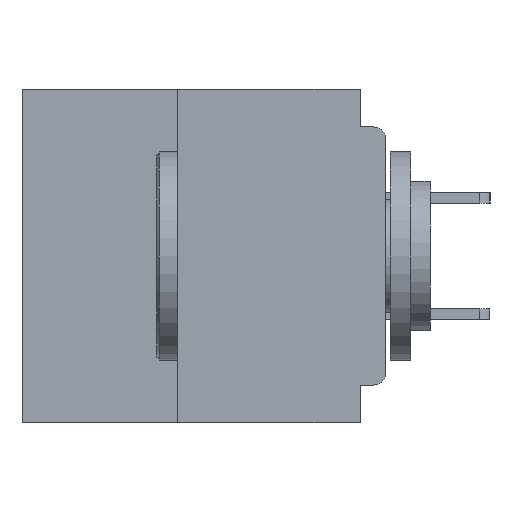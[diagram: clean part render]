
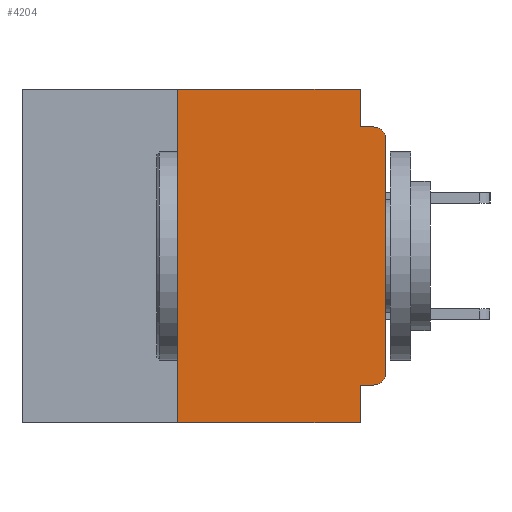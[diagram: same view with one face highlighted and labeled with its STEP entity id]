
A CAD part, left-side view. The second image highlights one B-rep face of the part: STEP entity #4204.
In plain terms, the highlighted planar face has unit normal (-1, 0, 0).
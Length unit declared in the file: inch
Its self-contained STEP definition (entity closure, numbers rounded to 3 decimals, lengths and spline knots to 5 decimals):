
#66 = VECTOR ( 'NONE', #5726, 39.37008 ) ;
#477 = ORIENTED_EDGE ( 'NONE', *, *, #27750, .T. ) ;
#1246 = LINE ( 'NONE', #16728, #11115 ) ;
#1715 = DIRECTION ( 'NONE',  ( 0., 0., -1. ) ) ;
#1983 = CARTESIAN_POINT ( 'NONE',  ( 0., 0., -0.045 ) ) ;
#2446 = CARTESIAN_POINT ( 'NONE',  ( 0., 0.015, -0.34 ) ) ;
#2610 = PLANE ( 'NONE',  #32171 ) ;
#2811 = EDGE_CURVE ( 'NONE', #2986, #11895, #3946, .T. ) ;
#2986 = VERTEX_POINT ( 'NONE', #45471 ) ;
#3946 = LINE ( 'NONE', #13473, #12645 ) ;
#3981 = ORIENTED_EDGE ( 'NONE', *, *, #2811, .F. ) ;
#4070 = CIRCLE ( 'NONE', #30709, 0.015 ) ;
#4204 = ADVANCED_FACE ( 'NONE', ( #39457 ), #2610, .F. ) ;
#5159 = ORIENTED_EDGE ( 'NONE', *, *, #5538, .F. ) ;
#5538 = EDGE_CURVE ( 'NONE', #42460, #2986, #29608, .T. ) ;
#5726 = DIRECTION ( 'NONE',  ( 0., -1., 0. ) ) ;
#6201 = DIRECTION ( 'NONE',  ( 0., 0., -1. ) ) ;
#6275 = ORIENTED_EDGE ( 'NONE', *, *, #23283, .F. ) ;
#6355 = DIRECTION ( 'NONE',  ( 1., 0., 0. ) ) ;
#6755 = EDGE_CURVE ( 'NONE', #13888, #23296, #25485, .T. ) ;
#8446 = LINE ( 'NONE', #23642, #26882 ) ;
#10859 = ORIENTED_EDGE ( 'NONE', *, *, #11515, .F. ) ;
#11115 = VECTOR ( 'NONE', #35025, 39.37008 ) ;
#11515 = EDGE_CURVE ( 'NONE', #15587, #40339, #39243, .T. ) ;
#11659 = DIRECTION ( 'NONE',  ( 0., 0., -1. ) ) ;
#11895 = VERTEX_POINT ( 'NONE', #29669 ) ;
#12645 = VECTOR ( 'NONE', #11659, 39.37008 ) ;
#12941 = VECTOR ( 'NONE', #17862, 39.37008 ) ;
#13473 = CARTESIAN_POINT ( 'NONE',  ( 0., 0.031, -0.4 ) ) ;
#13888 = VERTEX_POINT ( 'NONE', #44891 ) ;
#14512 = EDGE_CURVE ( 'NONE', #21854, #15587, #8446, .T. ) ;
#15587 = VERTEX_POINT ( 'NONE', #29735 ) ;
#16728 = CARTESIAN_POINT ( 'NONE',  ( 0., 0.25, -0.4 ) ) ;
#17862 = DIRECTION ( 'NONE',  ( 0., -1., 0. ) ) ;
#18737 = VECTOR ( 'NONE', #28932, 39.37008 ) ;
#21364 = VECTOR ( 'NONE', #36118, 39.37008 ) ;
#21854 = VERTEX_POINT ( 'NONE', #30813 ) ;
#21894 = VERTEX_POINT ( 'NONE', #45613 ) ;
#21908 = ORIENTED_EDGE ( 'NONE', *, *, #47481, .F. ) ;
#22548 = ORIENTED_EDGE ( 'NONE', *, *, #40474, .T. ) ;
#23283 = EDGE_CURVE ( 'NONE', #21894, #21854, #23938, .T. ) ;
#23296 = VERTEX_POINT ( 'NONE', #29077 ) ;
#23639 = CARTESIAN_POINT ( 'NONE',  ( 0., 0.25, -0.4 ) ) ;
#23642 = CARTESIAN_POINT ( 'NONE',  ( 0., 0.031, 0. ) ) ;
#23883 = DIRECTION ( 'NONE',  ( -1., 0., 0. ) ) ;
#23938 = LINE ( 'NONE', #47072, #12941 ) ;
#24154 = ORIENTED_EDGE ( 'NONE', *, *, #14512, .F. ) ;
#24997 = CARTESIAN_POINT ( 'NONE',  ( 0., 0., 0. ) ) ;
#25485 = LINE ( 'NONE', #24997, #43751 ) ;
#25825 = ORIENTED_EDGE ( 'NONE', *, *, #6755, .T. ) ;
#26882 = VECTOR ( 'NONE', #45294, 39.37008 ) ;
#27337 = EDGE_CURVE ( 'NONE', #23296, #40339, #30491, .T. ) ;
#27750 = EDGE_CURVE ( 'NONE', #42325, #11895, #40779, .T. ) ;
#28062 = CARTESIAN_POINT ( 'NONE',  ( 0., 0.015, -0.355 ) ) ;
#28242 = DIRECTION ( 'NONE',  ( -1., 0., 0. ) ) ;
#28655 = DIRECTION ( 'NONE',  ( 0., 0., 1. ) ) ;
#28932 = DIRECTION ( 'NONE',  ( 0., 1., 0. ) ) ;
#29077 = CARTESIAN_POINT ( 'NONE',  ( 0., 0., -0.06 ) ) ;
#29608 = LINE ( 'NONE', #47084, #18737 ) ;
#29669 = CARTESIAN_POINT ( 'NONE',  ( 0., 0.031, -0.4 ) ) ;
#29735 = CARTESIAN_POINT ( 'NONE',  ( 0., 0.031, -0.045 ) ) ;
#30491 = CIRCLE ( 'NONE', #47181, 0.015 ) ;
#30709 = AXIS2_PLACEMENT_3D ( 'NONE', #2446, #28242, #6201 ) ;
#30813 = CARTESIAN_POINT ( 'NONE',  ( 0., 0.031, 0. ) ) ;
#31152 = CARTESIAN_POINT ( 'NONE',  ( 0., 0.015, -0.045 ) ) ;
#31285 = EDGE_LOOP ( 'NONE', ( #25825, #38980, #10859, #24154, #6275, #21908, #477, #3981, #5159, #22548 ) ) ;
#32086 = DIRECTION ( 'NONE',  ( 0., 0., -1. ) ) ;
#32171 = AXIS2_PLACEMENT_3D ( 'NONE', #42919, #6355, #32086 ) ;
#35025 = DIRECTION ( 'NONE',  ( 0., 0., 1. ) ) ;
#36118 = DIRECTION ( 'NONE',  ( 0., -1., 0. ) ) ;
#38980 = ORIENTED_EDGE ( 'NONE', *, *, #27337, .T. ) ;
#39243 = LINE ( 'NONE', #1983, #66 ) ;
#39457 = FACE_OUTER_BOUND ( 'NONE', #31285, .T. ) ;
#39783 = CARTESIAN_POINT ( 'NONE',  ( 0., 0.437, -0.4 ) ) ;
#40339 = VERTEX_POINT ( 'NONE', #31152 ) ;
#40474 = EDGE_CURVE ( 'NONE', #42460, #13888, #4070, .T. ) ;
#40779 = LINE ( 'NONE', #39783, #21364 ) ;
#42325 = VERTEX_POINT ( 'NONE', #23639 ) ;
#42460 = VERTEX_POINT ( 'NONE', #28062 ) ;
#42919 = CARTESIAN_POINT ( 'NONE',  ( 0., 0.437, 0. ) ) ;
#43751 = VECTOR ( 'NONE', #28655, 39.37008 ) ;
#44891 = CARTESIAN_POINT ( 'NONE',  ( 0., 0., -0.34 ) ) ;
#45294 = DIRECTION ( 'NONE',  ( 0., 0., -1. ) ) ;
#45471 = CARTESIAN_POINT ( 'NONE',  ( 0., 0.031, -0.355 ) ) ;
#45613 = CARTESIAN_POINT ( 'NONE',  ( 0., 0.25, 0. ) ) ;
#45692 = CARTESIAN_POINT ( 'NONE',  ( 0., 0.015, -0.06 ) ) ;
#47072 = CARTESIAN_POINT ( 'NONE',  ( 0., 0.437, 0. ) ) ;
#47084 = CARTESIAN_POINT ( 'NONE',  ( 0., 0., -0.355 ) ) ;
#47181 = AXIS2_PLACEMENT_3D ( 'NONE', #45692, #23883, #1715 ) ;
#47481 = EDGE_CURVE ( 'NONE', #42325, #21894, #1246, .T. ) ;
